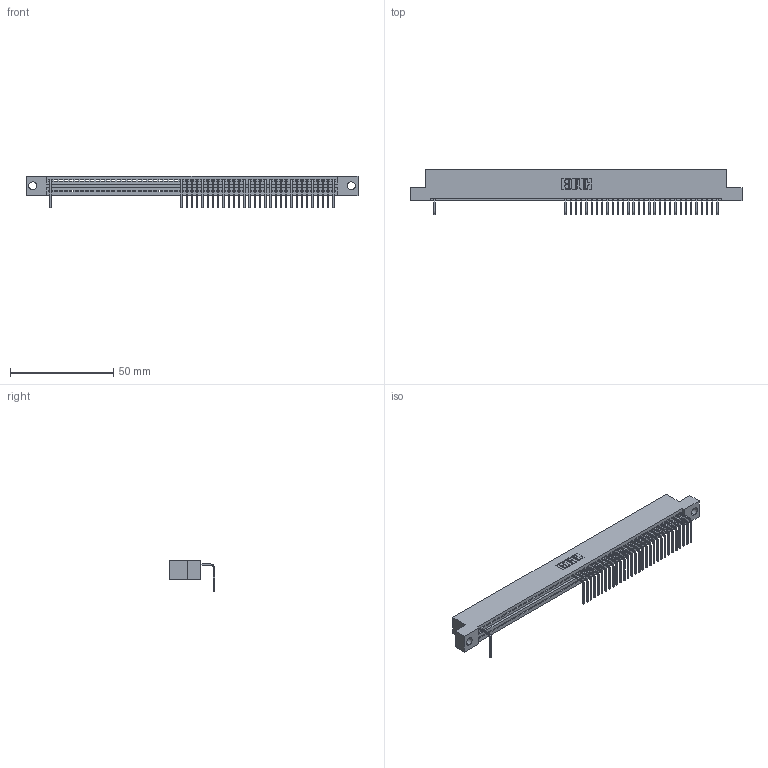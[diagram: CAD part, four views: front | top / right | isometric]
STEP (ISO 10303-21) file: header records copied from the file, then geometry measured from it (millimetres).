
FILE_DESCRIPTION (( 'STEP AP203' ), '1' );
FILE_NAME ('345-055-558-104.STEP', '2018-09-24T05:26:29', ( '' ), ( '' ), 'SwSTEP 2.0', 'SolidWorks 2016', '' );
FILE_SCHEMA (( 'CONFIG_CONTROL_DESIGN' ));
Length unit declared in the file: inch
Products named in the file (3): 345 Part_Flush Mounting Lugs - 0.156 Dia-TH; 345-292-001_558 Tail - 2; 345-055-558-104
Assembly tree (32 placements, depth 2):
  345-055-558-104
    345 Part_Flush Mounting Lugs - 0.156 Dia-TH
    345-292-001_558 Tail - 2  x31
Bounding box: 160.91 x 21.83 x 15.37 mm (x, y, z)
Volume: 15130.4 mm3; surface area: 19239.9 mm2
Topology: 32 solids, 32 shells, 2370 faces, 7279 edges, 4810 vertices
Faces by surface type: plane 1718, cylinder 652
Entity records: 38963 total; most frequent: ORIENTED_EDGE 6878, CARTESIAN_POINT 6865, DIRECTION 5949, EDGE_CURVE 3439, VECTOR 3087, LINE 3087, VERTEX_POINT 2290, AXIS2_PLACEMENT_3D 1431
